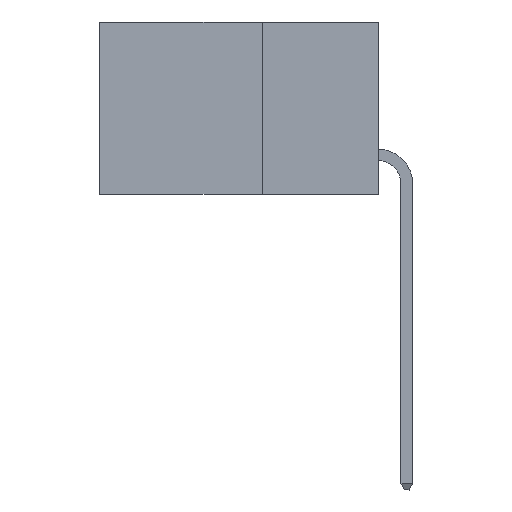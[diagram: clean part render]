
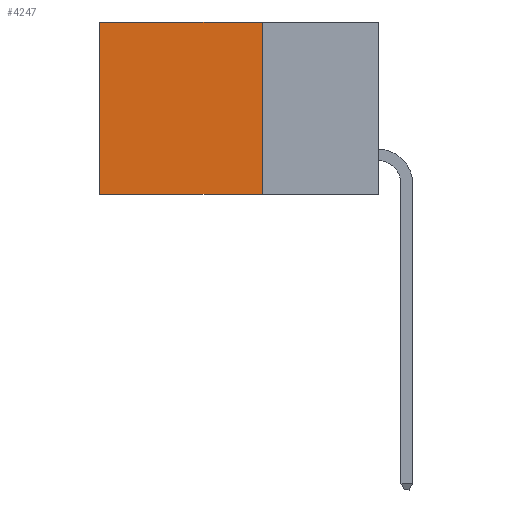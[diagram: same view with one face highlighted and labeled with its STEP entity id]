
A CAD part, left-side view. The second image highlights one B-rep face of the part: STEP entity #4247.
In plain terms, the highlighted planar face has unit normal (-1, 0, 0).
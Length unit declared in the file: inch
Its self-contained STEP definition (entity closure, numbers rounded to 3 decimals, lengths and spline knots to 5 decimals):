
#118 = DIRECTION ( 'NONE',  ( 0., 1., 0. ) ) ;
#968 = EDGE_LOOP ( 'NONE', ( #2565, #1694, #5094, #5291 ) ) ;
#1675 = VECTOR ( 'NONE', #118, 39.37008 ) ;
#1694 = ORIENTED_EDGE ( 'NONE', *, *, #10888, .F. ) ;
#1870 = VECTOR ( 'NONE', #6568, 39.37008 ) ;
#1999 = VECTOR ( 'NONE', #6362, 39.37008 ) ;
#2376 = EDGE_CURVE ( 'NONE', #3112, #5996, #11330, .T. ) ;
#2565 = ORIENTED_EDGE ( 'NONE', *, *, #9002, .T. ) ;
#3112 = VERTEX_POINT ( 'NONE', #8008 ) ;
#3190 = DIRECTION ( 'NONE',  ( 0., 0., -1. ) ) ;
#3209 = DIRECTION ( 'NONE',  ( 0., 0., -1. ) ) ;
#3338 = PLANE ( 'NONE',  #10309 ) ;
#4247 = ADVANCED_FACE ( 'NONE', ( #10835 ), #3338, .F. ) ;
#5094 = ORIENTED_EDGE ( 'NONE', *, *, #2376, .F. ) ;
#5291 = ORIENTED_EDGE ( 'NONE', *, *, #5847, .T. ) ;
#5454 = CARTESIAN_POINT ( 'NONE',  ( 0.298, 0.25, -0.37 ) ) ;
#5662 = VECTOR ( 'NONE', #3190, 39.37008 ) ;
#5847 = EDGE_CURVE ( 'NONE', #3112, #9520, #10928, .T. ) ;
#5996 = VERTEX_POINT ( 'NONE', #10789 ) ;
#6362 = DIRECTION ( 'NONE',  ( 0., 1., 0. ) ) ;
#6568 = DIRECTION ( 'NONE',  ( 0., 0., -1. ) ) ;
#6604 = CARTESIAN_POINT ( 'NONE',  ( 0.298, 0.25, 0. ) ) ;
#6738 = CARTESIAN_POINT ( 'NONE',  ( 0.298, 0.25, 0. ) ) ;
#6755 = CARTESIAN_POINT ( 'NONE',  ( 0.298, 0.6, 0. ) ) ;
#8008 = CARTESIAN_POINT ( 'NONE',  ( 0.298, 0.25, 0. ) ) ;
#8257 = LINE ( 'NONE', #10314, #5662 ) ;
#8457 = DIRECTION ( 'NONE',  ( 1., 0., 0. ) ) ;
#9002 = EDGE_CURVE ( 'NONE', #9520, #10931, #8257, .T. ) ;
#9278 = LINE ( 'NONE', #5454, #1999 ) ;
#9520 = VERTEX_POINT ( 'NONE', #6755 ) ;
#9537 = CARTESIAN_POINT ( 'NONE',  ( 0.298, 0.25, 0. ) ) ;
#9881 = CARTESIAN_POINT ( 'NONE',  ( 0.298, 0.6, -0.37 ) ) ;
#10309 = AXIS2_PLACEMENT_3D ( 'NONE', #9537, #8457, #3209 ) ;
#10314 = CARTESIAN_POINT ( 'NONE',  ( 0.298, 0.6, 0. ) ) ;
#10789 = CARTESIAN_POINT ( 'NONE',  ( 0.298, 0.25, -0.37 ) ) ;
#10835 = FACE_OUTER_BOUND ( 'NONE', #968, .T. ) ;
#10888 = EDGE_CURVE ( 'NONE', #5996, #10931, #9278, .T. ) ;
#10928 = LINE ( 'NONE', #6738, #1675 ) ;
#10931 = VERTEX_POINT ( 'NONE', #9881 ) ;
#11330 = LINE ( 'NONE', #6604, #1870 ) ;
